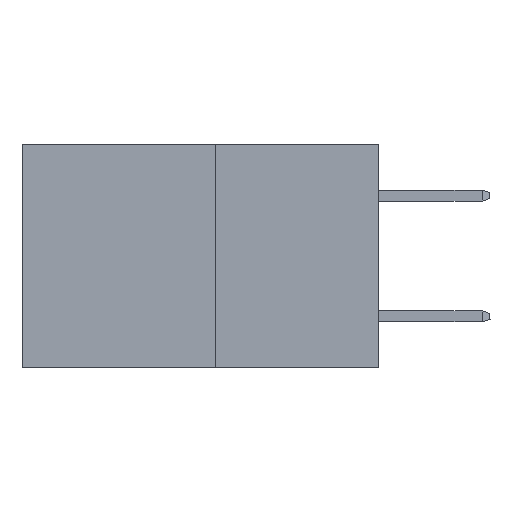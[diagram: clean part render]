
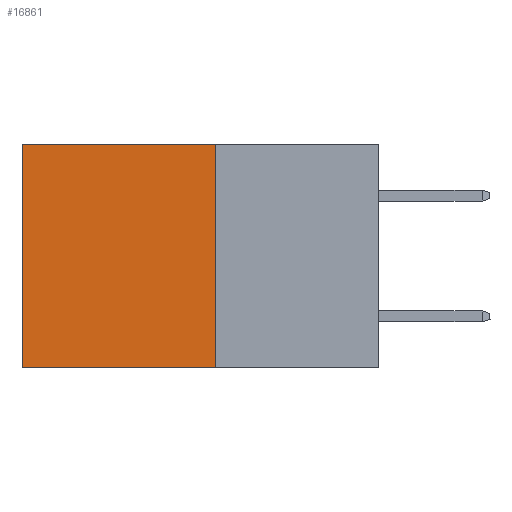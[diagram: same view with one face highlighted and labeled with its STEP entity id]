
A CAD part, left-side view. The second image highlights one B-rep face of the part: STEP entity #16861.
In plain terms, the highlighted planar face has unit normal (-1, 0, 0).
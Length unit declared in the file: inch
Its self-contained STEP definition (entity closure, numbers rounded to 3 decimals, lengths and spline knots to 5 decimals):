
#307 = VERTEX_POINT ( 'NONE', #24536 ) ;
#1081 = DIRECTION ( 'NONE',  ( 1., 0., 0. ) ) ;
#1364 = DIRECTION ( 'NONE',  ( 0., 0., -1. ) ) ;
#2691 = CARTESIAN_POINT ( 'NONE',  ( 0.277, 0.27, -0.37 ) ) ;
#2776 = CARTESIAN_POINT ( 'NONE',  ( 0.277, 0.27, 0. ) ) ;
#3380 = CARTESIAN_POINT ( 'NONE',  ( 0.277, 0.59, 0. ) ) ;
#3600 = EDGE_CURVE ( 'NONE', #8650, #6571, #23106, .T. ) ;
#3835 = LINE ( 'NONE', #2776, #9699 ) ;
#4205 = VECTOR ( 'NONE', #12998, 39.37008 ) ;
#4732 = EDGE_CURVE ( 'NONE', #307, #8650, #3835, .T. ) ;
#4993 = VERTEX_POINT ( 'NONE', #7974 ) ;
#5448 = VECTOR ( 'NONE', #1364, 39.37008 ) ;
#6224 = ORIENTED_EDGE ( 'NONE', *, *, #22712, .F. ) ;
#6571 = VERTEX_POINT ( 'NONE', #25152 ) ;
#6897 = FACE_OUTER_BOUND ( 'NONE', #15530, .T. ) ;
#7576 = AXIS2_PLACEMENT_3D ( 'NONE', #20940, #1081, #16561 ) ;
#7676 = PLANE ( 'NONE',  #7576 ) ;
#7974 = CARTESIAN_POINT ( 'NONE',  ( 0.277, 0.27, -0.37 ) ) ;
#8650 = VERTEX_POINT ( 'NONE', #3380 ) ;
#9371 = LINE ( 'NONE', #26316, #4205 ) ;
#9699 = VECTOR ( 'NONE', #18255, 39.37008 ) ;
#12998 = DIRECTION ( 'NONE',  ( 0., 0., -1. ) ) ;
#15530 = EDGE_LOOP ( 'NONE', ( #24822, #6224, #26276, #27062 ) ) ;
#16561 = DIRECTION ( 'NONE',  ( 0., 0., -1. ) ) ;
#16861 = ADVANCED_FACE ( 'NONE', ( #6897 ), #7676, .F. ) ;
#18173 = DIRECTION ( 'NONE',  ( 0., 1., 0. ) ) ;
#18255 = DIRECTION ( 'NONE',  ( 0., 1., 0. ) ) ;
#20359 = VECTOR ( 'NONE', #18173, 39.37008 ) ;
#20940 = CARTESIAN_POINT ( 'NONE',  ( 0.277, 0.27, -0.37 ) ) ;
#22467 = EDGE_CURVE ( 'NONE', #307, #4993, #9371, .T. ) ;
#22712 = EDGE_CURVE ( 'NONE', #4993, #6571, #25566, .T. ) ;
#23106 = LINE ( 'NONE', #27870, #5448 ) ;
#24536 = CARTESIAN_POINT ( 'NONE',  ( 0.277, 0.27, 0. ) ) ;
#24822 = ORIENTED_EDGE ( 'NONE', *, *, #3600, .T. ) ;
#25152 = CARTESIAN_POINT ( 'NONE',  ( 0.277, 0.59, -0.37 ) ) ;
#25566 = LINE ( 'NONE', #2691, #20359 ) ;
#26276 = ORIENTED_EDGE ( 'NONE', *, *, #22467, .F. ) ;
#26316 = CARTESIAN_POINT ( 'NONE',  ( 0.277, 0.27, -0.37 ) ) ;
#27062 = ORIENTED_EDGE ( 'NONE', *, *, #4732, .T. ) ;
#27870 = CARTESIAN_POINT ( 'NONE',  ( 0.277, 0.59, -0.37 ) ) ;
